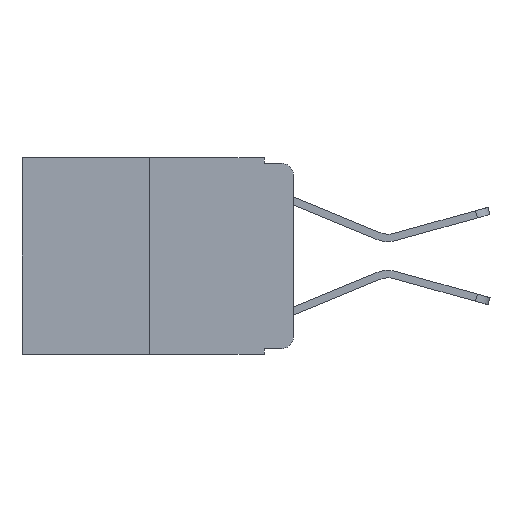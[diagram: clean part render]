
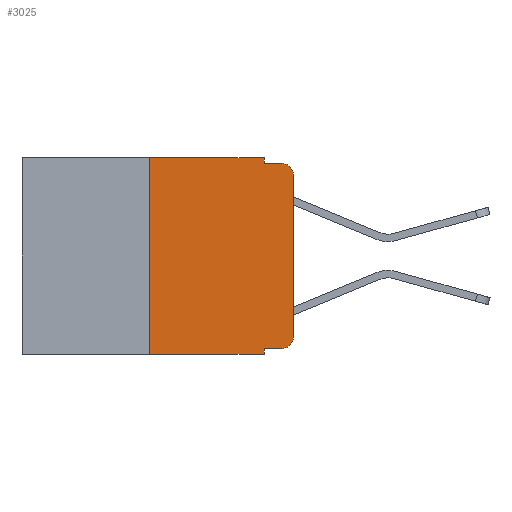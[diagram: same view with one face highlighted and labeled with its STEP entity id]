
A CAD part, left-side view. The second image highlights one B-rep face of the part: STEP entity #3025.
In plain terms, the highlighted planar face has unit normal (-1, 0, 0).
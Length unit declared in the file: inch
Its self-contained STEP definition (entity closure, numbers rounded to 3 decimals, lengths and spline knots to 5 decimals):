
#206 = CARTESIAN_POINT ( 'NONE',  ( 0., 0.051, 0. ) ) ;
#442 = CIRCLE ( 'NONE', #3227, 0.02 ) ;
#487 = DIRECTION ( 'NONE',  ( 0., -1., 0. ) ) ;
#517 = CARTESIAN_POINT ( 'NONE',  ( 0., 0.051, -0.01 ) ) ;
#611 = EDGE_CURVE ( 'NONE', #1861, #19158, #5851, .T. ) ;
#826 = AXIS2_PLACEMENT_3D ( 'NONE', #17468, #11467, #3445 ) ;
#987 = VECTOR ( 'NONE', #487, 39.37008 ) ;
#1126 = EDGE_CURVE ( 'NONE', #8066, #5256, #2176, .T. ) ;
#1861 = VERTEX_POINT ( 'NONE', #517 ) ;
#2176 = LINE ( 'NONE', #8713, #5836 ) ;
#3002 = VERTEX_POINT ( 'NONE', #17256 ) ;
#3025 = ADVANCED_FACE ( 'NONE', ( #4534 ), #12693, .F. ) ;
#3158 = CARTESIAN_POINT ( 'NONE',  ( 0., 0.473, 0. ) ) ;
#3227 = AXIS2_PLACEMENT_3D ( 'NONE', #6921, #6642, #6712 ) ;
#3293 = DIRECTION ( 'NONE',  ( 0., 0., -1. ) ) ;
#3445 = DIRECTION ( 'NONE',  ( 0., 0., -1. ) ) ;
#4026 = CARTESIAN_POINT ( 'NONE',  ( 0., 0.25, 0. ) ) ;
#4079 = DIRECTION ( 'NONE',  ( 0., -1., 0. ) ) ;
#4389 = VECTOR ( 'NONE', #13159, 39.37008 ) ;
#4424 = ORIENTED_EDGE ( 'NONE', *, *, #11364, .T. ) ;
#4534 = FACE_OUTER_BOUND ( 'NONE', #10645, .T. ) ;
#5256 = VERTEX_POINT ( 'NONE', #7856 ) ;
#5836 = VECTOR ( 'NONE', #4079, 39.37008 ) ;
#5851 = LINE ( 'NONE', #10923, #18823 ) ;
#6094 = EDGE_CURVE ( 'NONE', #8093, #1861, #9576, .T. ) ;
#6327 = CARTESIAN_POINT ( 'NONE',  ( 0., 0.051, 0. ) ) ;
#6334 = DIRECTION ( 'NONE',  ( 1., 0., 0. ) ) ;
#6505 = CARTESIAN_POINT ( 'NONE',  ( 0., 0., -0.03 ) ) ;
#6554 = LINE ( 'NONE', #8040, #11951 ) ;
#6642 = DIRECTION ( 'NONE',  ( -1., 0., 0. ) ) ;
#6672 = CARTESIAN_POINT ( 'NONE',  ( 0., 0., -0.313 ) ) ;
#6712 = DIRECTION ( 'NONE',  ( 0., 0., -1. ) ) ;
#6746 = CARTESIAN_POINT ( 'NONE',  ( 0., 0.473, 0. ) ) ;
#6854 = CARTESIAN_POINT ( 'NONE',  ( 0., 0.25, -0.343 ) ) ;
#6921 = CARTESIAN_POINT ( 'NONE',  ( 0., 0.02, -0.313 ) ) ;
#7055 = VERTEX_POINT ( 'NONE', #4026 ) ;
#7226 = VERTEX_POINT ( 'NONE', #6505 ) ;
#7856 = CARTESIAN_POINT ( 'NONE',  ( 0., 0.051, -0.343 ) ) ;
#8040 = CARTESIAN_POINT ( 'NONE',  ( 0., 0.25, 0. ) ) ;
#8066 = VERTEX_POINT ( 'NONE', #6854 ) ;
#8093 = VERTEX_POINT ( 'NONE', #17890 ) ;
#8143 = ORIENTED_EDGE ( 'NONE', *, *, #6094, .F. ) ;
#8569 = ORIENTED_EDGE ( 'NONE', *, *, #18726, .F. ) ;
#8713 = CARTESIAN_POINT ( 'NONE',  ( 0., 0.473, -0.343 ) ) ;
#9331 = EDGE_CURVE ( 'NONE', #15248, #7226, #14426, .T. ) ;
#9488 = DIRECTION ( 'NONE',  ( 0., 0., -1. ) ) ;
#9520 = CARTESIAN_POINT ( 'NONE',  ( 0., 0.02, -0.01 ) ) ;
#9576 = LINE ( 'NONE', #6327, #12758 ) ;
#10145 = ORIENTED_EDGE ( 'NONE', *, *, #14063, .T. ) ;
#10203 = EDGE_CURVE ( 'NONE', #8066, #7055, #6554, .T. ) ;
#10217 = EDGE_CURVE ( 'NONE', #14933, #5256, #18561, .T. ) ;
#10645 = EDGE_LOOP ( 'NONE', ( #15804, #4424, #16970, #8143, #8569, #18512, #11139, #13268, #15502, #10145 ) ) ;
#10923 = CARTESIAN_POINT ( 'NONE',  ( 0., 0.051, -0.01 ) ) ;
#11139 = ORIENTED_EDGE ( 'NONE', *, *, #1126, .T. ) ;
#11364 = EDGE_CURVE ( 'NONE', #7226, #19158, #18610, .T. ) ;
#11467 = DIRECTION ( 'NONE',  ( -1., 0., 0. ) ) ;
#11951 = VECTOR ( 'NONE', #14752, 39.37008 ) ;
#12091 = CARTESIAN_POINT ( 'NONE',  ( 0., 0.051, -0.333 ) ) ;
#12265 = LINE ( 'NONE', #6746, #12759 ) ;
#12693 = PLANE ( 'NONE',  #16978 ) ;
#12706 = EDGE_CURVE ( 'NONE', #14933, #3002, #18591, .T. ) ;
#12758 = VECTOR ( 'NONE', #3293, 39.37008 ) ;
#12759 = VECTOR ( 'NONE', #19014, 39.37008 ) ;
#13159 = DIRECTION ( 'NONE',  ( 0., 0., -1. ) ) ;
#13268 = ORIENTED_EDGE ( 'NONE', *, *, #10217, .F. ) ;
#14063 = EDGE_CURVE ( 'NONE', #3002, #15248, #442, .T. ) ;
#14426 = LINE ( 'NONE', #18552, #15665 ) ;
#14752 = DIRECTION ( 'NONE',  ( 0., 0., 1. ) ) ;
#14933 = VERTEX_POINT ( 'NONE', #12091 ) ;
#15248 = VERTEX_POINT ( 'NONE', #6672 ) ;
#15502 = ORIENTED_EDGE ( 'NONE', *, *, #12706, .T. ) ;
#15665 = VECTOR ( 'NONE', #18689, 39.37008 ) ;
#15804 = ORIENTED_EDGE ( 'NONE', *, *, #9331, .T. ) ;
#16970 = ORIENTED_EDGE ( 'NONE', *, *, #611, .F. ) ;
#16978 = AXIS2_PLACEMENT_3D ( 'NONE', #3158, #6334, #9488 ) ;
#17256 = CARTESIAN_POINT ( 'NONE',  ( 0., 0.02, -0.333 ) ) ;
#17468 = CARTESIAN_POINT ( 'NONE',  ( 0., 0.02, -0.03 ) ) ;
#17890 = CARTESIAN_POINT ( 'NONE',  ( 0., 0.051, 0. ) ) ;
#18464 = DIRECTION ( 'NONE',  ( 0., -1., 0. ) ) ;
#18512 = ORIENTED_EDGE ( 'NONE', *, *, #10203, .F. ) ;
#18552 = CARTESIAN_POINT ( 'NONE',  ( 0., 0., 0. ) ) ;
#18561 = LINE ( 'NONE', #206, #4389 ) ;
#18591 = LINE ( 'NONE', #19164, #987 ) ;
#18610 = CIRCLE ( 'NONE', #826, 0.02 ) ;
#18689 = DIRECTION ( 'NONE',  ( 0., 0., 1. ) ) ;
#18726 = EDGE_CURVE ( 'NONE', #7055, #8093, #12265, .T. ) ;
#18823 = VECTOR ( 'NONE', #18464, 39.37008 ) ;
#19014 = DIRECTION ( 'NONE',  ( 0., -1., 0. ) ) ;
#19158 = VERTEX_POINT ( 'NONE', #9520 ) ;
#19164 = CARTESIAN_POINT ( 'NONE',  ( 0., 0.051, -0.333 ) ) ;
